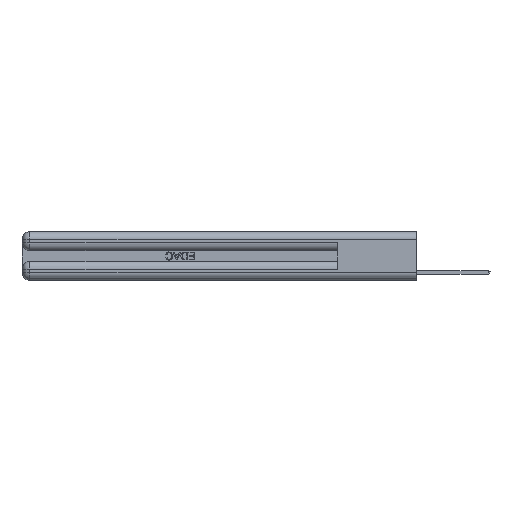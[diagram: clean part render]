
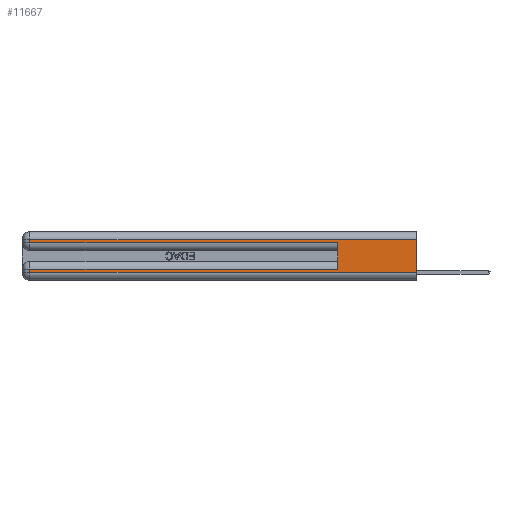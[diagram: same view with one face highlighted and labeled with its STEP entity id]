
A CAD part, left-side view. The second image highlights one B-rep face of the part: STEP entity #11667.
In plain terms, the highlighted planar face has unit normal (-1, 0, 0).
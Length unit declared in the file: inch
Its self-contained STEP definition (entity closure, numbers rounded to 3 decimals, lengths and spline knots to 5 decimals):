
#641 = EDGE_CURVE ( 'NONE', #21108, #25045, #30164, .T. ) ;
#680 = DIRECTION ( 'NONE',  ( 0., 0., -1. ) ) ;
#950 = VERTEX_POINT ( 'NONE', #15943 ) ;
#1238 = ORIENTED_EDGE ( 'NONE', *, *, #12335, .T. ) ;
#1400 = DIRECTION ( 'NONE',  ( 0., 0., -1. ) ) ;
#2019 = LINE ( 'NONE', #22707, #9534 ) ;
#2839 = CARTESIAN_POINT ( 'NONE',  ( 0., 0., 0.31 ) ) ;
#3292 = EDGE_CURVE ( 'NONE', #7312, #11583, #8569, .T. ) ;
#3600 = ORIENTED_EDGE ( 'NONE', *, *, #18646, .F. ) ;
#4265 = AXIS2_PLACEMENT_3D ( 'NONE', #16201, #16639, #1400 ) ;
#4560 = CARTESIAN_POINT ( 'NONE',  ( 0., 2.94, 0.37 ) ) ;
#4629 = CARTESIAN_POINT ( 'NONE',  ( 0., 0., 0.085 ) ) ;
#4910 = VERTEX_POINT ( 'NONE', #8414 ) ;
#5577 = VECTOR ( 'NONE', #9578, 39.37008 ) ;
#6955 = CARTESIAN_POINT ( 'NONE',  ( 0., 0., 0.31 ) ) ;
#7312 = VERTEX_POINT ( 'NONE', #21856 ) ;
#8414 = CARTESIAN_POINT ( 'NONE',  ( 0., 0.6, 0.085 ) ) ;
#8569 = LINE ( 'NONE', #4560, #25168 ) ;
#9004 = ORIENTED_EDGE ( 'NONE', *, *, #20473, .F. ) ;
#9534 = VECTOR ( 'NONE', #10422, 39.37008 ) ;
#9578 = DIRECTION ( 'NONE',  ( 0., 1., 0. ) ) ;
#9699 = LINE ( 'NONE', #18357, #29056 ) ;
#10422 = DIRECTION ( 'NONE',  ( 0., 0., 1. ) ) ;
#11583 = VERTEX_POINT ( 'NONE', #18963 ) ;
#11667 = ADVANCED_FACE ( 'NONE', ( #11908 ), #26476, .F. ) ;
#11895 = VECTOR ( 'NONE', #31911, 39.37008 ) ;
#11908 = FACE_OUTER_BOUND ( 'NONE', #12709, .T. ) ;
#12297 = LINE ( 'NONE', #4629, #5577 ) ;
#12307 = EDGE_CURVE ( 'NONE', #25045, #21604, #14243, .T. ) ;
#12335 = EDGE_CURVE ( 'NONE', #11583, #950, #21742, .T. ) ;
#12709 = EDGE_LOOP ( 'NONE', ( #3600, #24525, #19731, #1238, #9004, #13489, #27286, #15945 ) ) ;
#13439 = VECTOR ( 'NONE', #26445, 39.37008 ) ;
#13489 = ORIENTED_EDGE ( 'NONE', *, *, #32269, .T. ) ;
#14179 = DIRECTION ( 'NONE',  ( 0., 0., -1. ) ) ;
#14243 = LINE ( 'NONE', #21469, #13439 ) ;
#15758 = CARTESIAN_POINT ( 'NONE',  ( 0., 2.94, 0.37 ) ) ;
#15943 = CARTESIAN_POINT ( 'NONE',  ( 0., 0.6, 0.285 ) ) ;
#15945 = ORIENTED_EDGE ( 'NONE', *, *, #12307, .T. ) ;
#16201 = CARTESIAN_POINT ( 'NONE',  ( 0., 0., 0.37 ) ) ;
#16639 = DIRECTION ( 'NONE',  ( 1., 0., 0. ) ) ;
#16947 = CARTESIAN_POINT ( 'NONE',  ( 0., 2.94, 0.06 ) ) ;
#18357 = CARTESIAN_POINT ( 'NONE',  ( 0., 0., 0.37 ) ) ;
#18646 = EDGE_CURVE ( 'NONE', #19836, #21604, #9699, .T. ) ;
#18963 = CARTESIAN_POINT ( 'NONE',  ( 0., 2.94, 0.285 ) ) ;
#19138 = CARTESIAN_POINT ( 'NONE',  ( 0., 0., 0.285 ) ) ;
#19494 = VECTOR ( 'NONE', #25922, 39.37008 ) ;
#19731 = ORIENTED_EDGE ( 'NONE', *, *, #3292, .T. ) ;
#19836 = VERTEX_POINT ( 'NONE', #2839 ) ;
#20449 = CARTESIAN_POINT ( 'NONE',  ( 0., 2.94, 0.085 ) ) ;
#20473 = EDGE_CURVE ( 'NONE', #4910, #950, #2019, .T. ) ;
#21108 = VERTEX_POINT ( 'NONE', #20449 ) ;
#21469 = CARTESIAN_POINT ( 'NONE',  ( 0., 0., 0.06 ) ) ;
#21604 = VERTEX_POINT ( 'NONE', #22192 ) ;
#21742 = LINE ( 'NONE', #19138, #24901 ) ;
#21856 = CARTESIAN_POINT ( 'NONE',  ( 0., 2.94, 0.31 ) ) ;
#22192 = CARTESIAN_POINT ( 'NONE',  ( 0., 0., 0.06 ) ) ;
#22707 = CARTESIAN_POINT ( 'NONE',  ( 0., 0.6, 0.145 ) ) ;
#24525 = ORIENTED_EDGE ( 'NONE', *, *, #32231, .T. ) ;
#24901 = VECTOR ( 'NONE', #28952, 39.37008 ) ;
#25045 = VERTEX_POINT ( 'NONE', #16947 ) ;
#25168 = VECTOR ( 'NONE', #14179, 39.37008 ) ;
#25922 = DIRECTION ( 'NONE',  ( 0., 0., -1. ) ) ;
#26445 = DIRECTION ( 'NONE',  ( 0., -1., 0. ) ) ;
#26476 = PLANE ( 'NONE',  #4265 ) ;
#27286 = ORIENTED_EDGE ( 'NONE', *, *, #641, .T. ) ;
#28952 = DIRECTION ( 'NONE',  ( 0., -1., 0. ) ) ;
#29056 = VECTOR ( 'NONE', #680, 39.37008 ) ;
#30164 = LINE ( 'NONE', #15758, #19494 ) ;
#31911 = DIRECTION ( 'NONE',  ( 0., 1., 0. ) ) ;
#32231 = EDGE_CURVE ( 'NONE', #19836, #7312, #32441, .T. ) ;
#32269 = EDGE_CURVE ( 'NONE', #4910, #21108, #12297, .T. ) ;
#32441 = LINE ( 'NONE', #6955, #11895 ) ;
